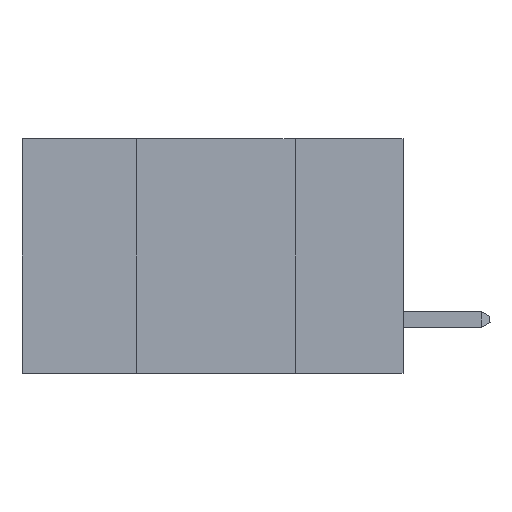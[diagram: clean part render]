
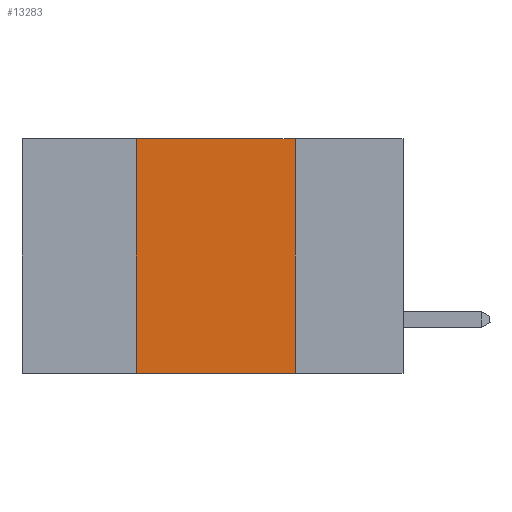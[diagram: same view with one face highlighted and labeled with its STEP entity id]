
A CAD part, left-side view. The second image highlights one B-rep face of the part: STEP entity #13283.
In plain terms, the highlighted planar face has unit normal (-1, 0, 0).
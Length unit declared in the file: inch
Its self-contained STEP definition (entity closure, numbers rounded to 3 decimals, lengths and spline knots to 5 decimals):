
#558 = VERTEX_POINT ( 'NONE', #10450 ) ;
#1298 = VECTOR ( 'NONE', #6377, 39.37008 ) ;
#2036 = LINE ( 'NONE', #7107, #5904 ) ;
#3339 = FACE_OUTER_BOUND ( 'NONE', #4107, .T. ) ;
#3482 = DIRECTION ( 'NONE',  ( 0., -1., 0. ) ) ;
#3714 = LINE ( 'NONE', #4717, #1298 ) ;
#3744 = EDGE_CURVE ( 'NONE', #16205, #5013, #2036, .T. ) ;
#3879 = LINE ( 'NONE', #18809, #20502 ) ;
#4107 = EDGE_LOOP ( 'NONE', ( #11049, #6957, #17824, #9389 ) ) ;
#4717 = CARTESIAN_POINT ( 'NONE',  ( 0., 0.6, 0. ) ) ;
#5013 = VERTEX_POINT ( 'NONE', #19541 ) ;
#5844 = CARTESIAN_POINT ( 'NONE',  ( 0., 0.6, 0. ) ) ;
#5904 = VECTOR ( 'NONE', #14666, 39.37008 ) ;
#6377 = DIRECTION ( 'NONE',  ( 0., -1., 0. ) ) ;
#6957 = ORIENTED_EDGE ( 'NONE', *, *, #24674, .F. ) ;
#7107 = CARTESIAN_POINT ( 'NONE',  ( 0., 0.17, 0. ) ) ;
#9389 = ORIENTED_EDGE ( 'NONE', *, *, #16167, .T. ) ;
#9810 = DIRECTION ( 'NONE',  ( 0., 0., -1. ) ) ;
#10450 = CARTESIAN_POINT ( 'NONE',  ( 0., 0.42, 0. ) ) ;
#10580 = AXIS2_PLACEMENT_3D ( 'NONE', #5844, #13226, #9810 ) ;
#11049 = ORIENTED_EDGE ( 'NONE', *, *, #3744, .F. ) ;
#13226 = DIRECTION ( 'NONE',  ( 1., 0., 0. ) ) ;
#13283 = ADVANCED_FACE ( 'NONE', ( #3339 ), #19137, .F. ) ;
#13428 = CARTESIAN_POINT ( 'NONE',  ( 0., 0.42, -0.37 ) ) ;
#14578 = LINE ( 'NONE', #16047, #20313 ) ;
#14666 = DIRECTION ( 'NONE',  ( 0., 0., -1. ) ) ;
#16047 = CARTESIAN_POINT ( 'NONE',  ( 0., 0.42, 0. ) ) ;
#16167 = EDGE_CURVE ( 'NONE', #20244, #5013, #3879, .T. ) ;
#16205 = VERTEX_POINT ( 'NONE', #22956 ) ;
#17824 = ORIENTED_EDGE ( 'NONE', *, *, #24591, .F. ) ;
#18164 = DIRECTION ( 'NONE',  ( 0., 0., 1. ) ) ;
#18809 = CARTESIAN_POINT ( 'NONE',  ( 0., 0.6, -0.37 ) ) ;
#19137 = PLANE ( 'NONE',  #10580 ) ;
#19541 = CARTESIAN_POINT ( 'NONE',  ( 0., 0.17, -0.37 ) ) ;
#20244 = VERTEX_POINT ( 'NONE', #13428 ) ;
#20313 = VECTOR ( 'NONE', #18164, 39.37008 ) ;
#20502 = VECTOR ( 'NONE', #3482, 39.37008 ) ;
#22956 = CARTESIAN_POINT ( 'NONE',  ( 0., 0.17, 0. ) ) ;
#24591 = EDGE_CURVE ( 'NONE', #20244, #558, #14578, .T. ) ;
#24674 = EDGE_CURVE ( 'NONE', #558, #16205, #3714, .T. ) ;
